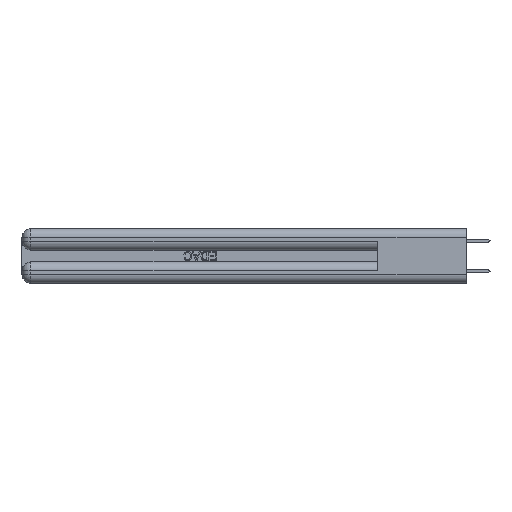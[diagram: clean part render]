
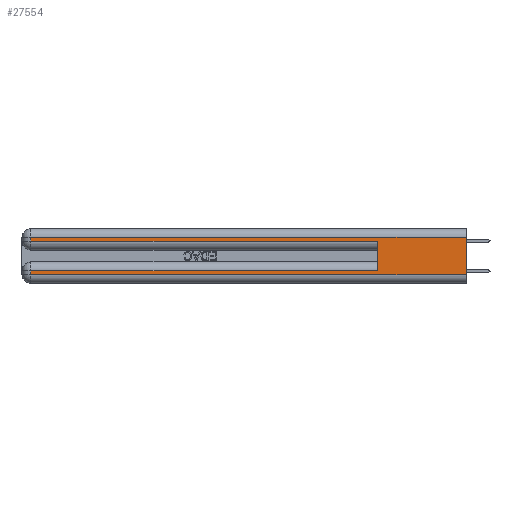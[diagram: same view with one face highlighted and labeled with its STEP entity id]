
A CAD part, left-side view. The second image highlights one B-rep face of the part: STEP entity #27554.
In plain terms, the highlighted planar face has unit normal (-1, 0, 0).
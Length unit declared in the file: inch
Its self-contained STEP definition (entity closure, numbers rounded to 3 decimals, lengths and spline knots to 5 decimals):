
#567 = VECTOR ( 'NONE', #31829, 39.37008 ) ;
#2485 = EDGE_CURVE ( 'NONE', #16957, #13184, #10063, .T. ) ;
#2496 = CARTESIAN_POINT ( 'NONE',  ( 0., 0., 0.31 ) ) ;
#2638 = VERTEX_POINT ( 'NONE', #36260 ) ;
#3430 = EDGE_LOOP ( 'NONE', ( #30875, #26836, #8454, #41217, #11813, #23707, #17854, #15108 ) ) ;
#3689 = VECTOR ( 'NONE', #34039, 39.37008 ) ;
#3725 = VERTEX_POINT ( 'NONE', #25672 ) ;
#3889 = VECTOR ( 'NONE', #22999, 39.37008 ) ;
#6238 = CARTESIAN_POINT ( 'NONE',  ( 0., 0., 0.06 ) ) ;
#6397 = CARTESIAN_POINT ( 'NONE',  ( 0., 2.94, 0.06 ) ) ;
#6920 = CARTESIAN_POINT ( 'NONE',  ( 0., 0., 0.285 ) ) ;
#7363 = CARTESIAN_POINT ( 'NONE',  ( 0., 2.94, 0.37 ) ) ;
#7553 = CARTESIAN_POINT ( 'NONE',  ( 0., 0.6, 0.085 ) ) ;
#8454 = ORIENTED_EDGE ( 'NONE', *, *, #39026, .T. ) ;
#9105 = EDGE_CURVE ( 'NONE', #16957, #2638, #23382, .T. ) ;
#9133 = LINE ( 'NONE', #6238, #567 ) ;
#9657 = EDGE_CURVE ( 'NONE', #33240, #3725, #21325, .T. ) ;
#10008 = CARTESIAN_POINT ( 'NONE',  ( 0., 0., 0.37 ) ) ;
#10063 = LINE ( 'NONE', #14218, #33586 ) ;
#10137 = DIRECTION ( 'NONE',  ( 1., 0., 0. ) ) ;
#10521 = CARTESIAN_POINT ( 'NONE',  ( 0., 2.94, 0.085 ) ) ;
#10862 = AXIS2_PLACEMENT_3D ( 'NONE', #10008, #10137, #32509 ) ;
#11238 = VECTOR ( 'NONE', #26536, 39.37008 ) ;
#11813 = ORIENTED_EDGE ( 'NONE', *, *, #9657, .F. ) ;
#12126 = VECTOR ( 'NONE', #28020, 39.37008 ) ;
#12181 = LINE ( 'NONE', #24243, #3689 ) ;
#13184 = VERTEX_POINT ( 'NONE', #27213 ) ;
#14218 = CARTESIAN_POINT ( 'NONE',  ( 0., 0., 0.31 ) ) ;
#14362 = DIRECTION ( 'NONE',  ( 0., 1., 0. ) ) ;
#15108 = ORIENTED_EDGE ( 'NONE', *, *, #15139, .T. ) ;
#15139 = EDGE_CURVE ( 'NONE', #39881, #2638, #9133, .T. ) ;
#16957 = VERTEX_POINT ( 'NONE', #2496 ) ;
#17700 = VERTEX_POINT ( 'NONE', #10521 ) ;
#17854 = ORIENTED_EDGE ( 'NONE', *, *, #33913, .T. ) ;
#20325 = VECTOR ( 'NONE', #40323, 39.37008 ) ;
#21325 = LINE ( 'NONE', #24368, #20325 ) ;
#21513 = CARTESIAN_POINT ( 'NONE',  ( 0., 2.94, 0.285 ) ) ;
#22359 = VECTOR ( 'NONE', #33765, 39.37008 ) ;
#22999 = DIRECTION ( 'NONE',  ( 0., -1., 0. ) ) ;
#23096 = VERTEX_POINT ( 'NONE', #21513 ) ;
#23382 = LINE ( 'NONE', #33501, #22359 ) ;
#23707 = ORIENTED_EDGE ( 'NONE', *, *, #23922, .T. ) ;
#23922 = EDGE_CURVE ( 'NONE', #33240, #17700, #30162, .T. ) ;
#24243 = CARTESIAN_POINT ( 'NONE',  ( 0., 2.94, 0.37 ) ) ;
#24368 = CARTESIAN_POINT ( 'NONE',  ( 0., 0.6, 0.145 ) ) ;
#25672 = CARTESIAN_POINT ( 'NONE',  ( 0., 0.6, 0.285 ) ) ;
#26536 = DIRECTION ( 'NONE',  ( 0., 0., -1. ) ) ;
#26836 = ORIENTED_EDGE ( 'NONE', *, *, #2485, .T. ) ;
#27213 = CARTESIAN_POINT ( 'NONE',  ( 0., 2.94, 0.31 ) ) ;
#27554 = ADVANCED_FACE ( 'NONE', ( #30413 ), #29285, .F. ) ;
#27560 = EDGE_CURVE ( 'NONE', #23096, #3725, #29401, .T. ) ;
#28020 = DIRECTION ( 'NONE',  ( 0., 1., 0. ) ) ;
#28259 = LINE ( 'NONE', #7363, #11238 ) ;
#29285 = PLANE ( 'NONE',  #10862 ) ;
#29401 = LINE ( 'NONE', #6920, #3889 ) ;
#30162 = LINE ( 'NONE', #37675, #12126 ) ;
#30413 = FACE_OUTER_BOUND ( 'NONE', #3430, .T. ) ;
#30875 = ORIENTED_EDGE ( 'NONE', *, *, #9105, .F. ) ;
#31829 = DIRECTION ( 'NONE',  ( 0., -1., 0. ) ) ;
#32509 = DIRECTION ( 'NONE',  ( 0., 0., -1. ) ) ;
#33240 = VERTEX_POINT ( 'NONE', #7553 ) ;
#33501 = CARTESIAN_POINT ( 'NONE',  ( 0., 0., 0.37 ) ) ;
#33586 = VECTOR ( 'NONE', #14362, 39.37008 ) ;
#33765 = DIRECTION ( 'NONE',  ( 0., 0., -1. ) ) ;
#33913 = EDGE_CURVE ( 'NONE', #17700, #39881, #28259, .T. ) ;
#34039 = DIRECTION ( 'NONE',  ( 0., 0., -1. ) ) ;
#36260 = CARTESIAN_POINT ( 'NONE',  ( 0., 0., 0.06 ) ) ;
#37675 = CARTESIAN_POINT ( 'NONE',  ( 0., 0., 0.085 ) ) ;
#39026 = EDGE_CURVE ( 'NONE', #13184, #23096, #12181, .T. ) ;
#39881 = VERTEX_POINT ( 'NONE', #6397 ) ;
#40323 = DIRECTION ( 'NONE',  ( 0., 0., 1. ) ) ;
#41217 = ORIENTED_EDGE ( 'NONE', *, *, #27560, .T. ) ;
